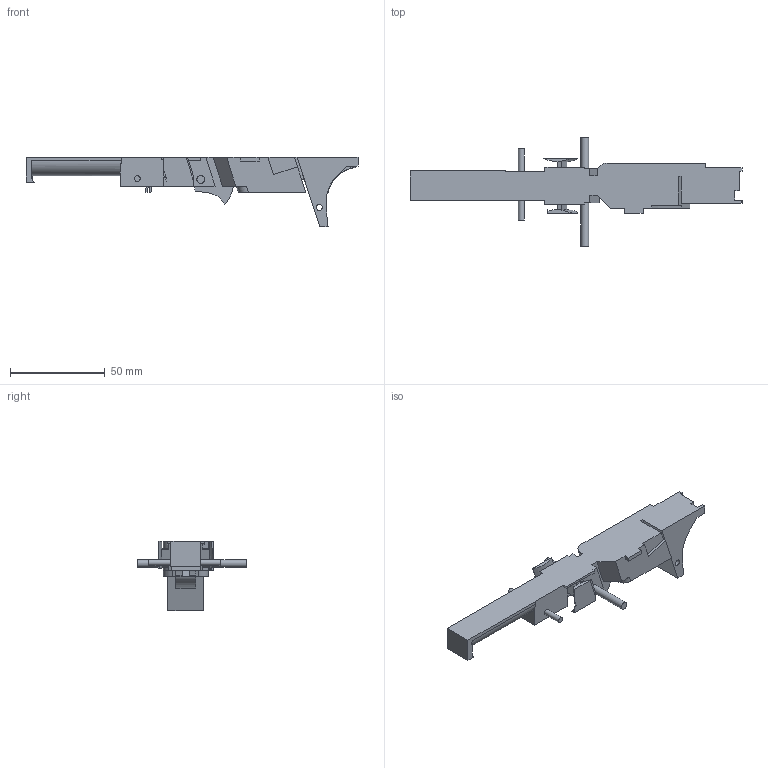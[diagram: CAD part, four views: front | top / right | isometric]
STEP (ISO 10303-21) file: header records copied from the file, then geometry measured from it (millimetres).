
FILE_DESCRIPTION(/* description */ (''),/* implementation_level */ '2;1');
FILE_NAME(/* name */ 'py2a_g19_control_negative v1.step',/* time_stamp */ '2021-09-02T09:00:33-05:00',/* author */ (''),/* organization */ (''),/* preprocessor_version */ 'ST-DEVELOPER v18.1',/* originating_system */ 'Autodesk Translation Framework v10.10.0.1391',/* authorisation */ '');
FILE_SCHEMA (('AUTOMOTIVE_DESIGN { 1 0 10303 214 3 1 1 }'));
Length unit declared in the file: millimetre
Products named in the file (2): py2a_g19_control_negative; G19ControlPocket
Assembly tree (1 placements, depth 2):
  py2a_g19_control_negative
    G19ControlPocket
Bounding box: 175 x 57.44 x 36.54 mm (x, y, z)
Volume: 47029.4 mm3; surface area: 16341.8 mm2
Topology: 1 solids, 1 shells, 160 faces, 446 edges, 296 vertices
Faces by surface type: plane 127, bspline 17, cylinder 16
Full cylindrical faces by diameter (mm): 3.05 x2, 3.147 x1, 4.1 x2
Entity records: 7102 total; most frequent: CARTESIAN_POINT 3028, ORIENTED_EDGE 892, DIRECTION 740, EDGE_CURVE 446, LINE 350, VECTOR 350, VERTEX_POINT 296, AXIS2_PLACEMENT_3D 195
